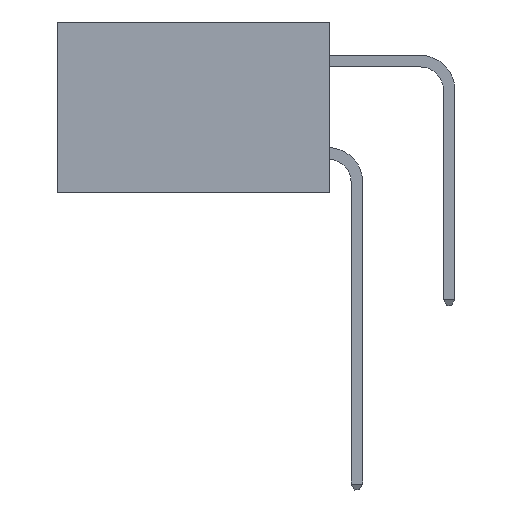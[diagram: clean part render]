
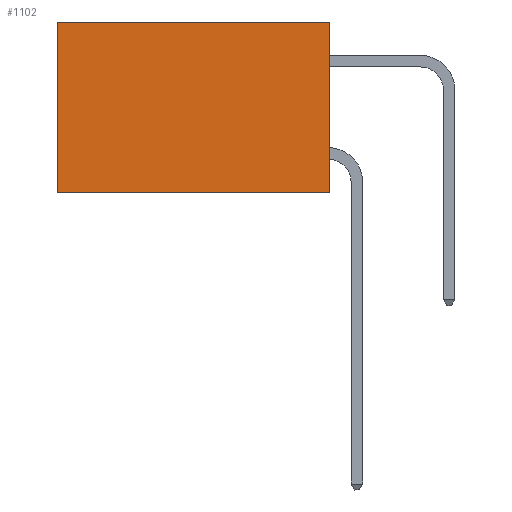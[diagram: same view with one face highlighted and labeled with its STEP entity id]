
A CAD part, left-side view. The second image highlights one B-rep face of the part: STEP entity #1102.
In plain terms, the highlighted planar face has unit normal (-1, 0, 0).
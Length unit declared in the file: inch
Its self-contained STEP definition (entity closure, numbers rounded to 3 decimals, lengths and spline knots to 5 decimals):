
#195 = AXIS2_PLACEMENT_3D ( 'NONE', #9011, #692, #2740 ) ;
#692 = DIRECTION ( 'NONE',  ( 1., 0., 0. ) ) ;
#1022 = DIRECTION ( 'NONE',  ( 0., 0., -1. ) ) ;
#1102 = ADVANCED_FACE ( 'NONE', ( #3993 ), #2985, .F. ) ;
#1484 = CARTESIAN_POINT ( 'NONE',  ( 0.277, 0.59, -0.37 ) ) ;
#1709 = DIRECTION ( 'NONE',  ( 0., 1., 0. ) ) ;
#2141 = CARTESIAN_POINT ( 'NONE',  ( 0.277, 0., 0. ) ) ;
#2303 = LINE ( 'NONE', #5238, #6686 ) ;
#2310 = VERTEX_POINT ( 'NONE', #2141 ) ;
#2450 = VERTEX_POINT ( 'NONE', #1484 ) ;
#2740 = DIRECTION ( 'NONE',  ( 0., 0., -1. ) ) ;
#2827 = CARTESIAN_POINT ( 'NONE',  ( 0.277, 0., 0. ) ) ;
#2985 = PLANE ( 'NONE',  #195 ) ;
#3219 = LINE ( 'NONE', #6325, #5651 ) ;
#3993 = FACE_OUTER_BOUND ( 'NONE', #5499, .T. ) ;
#5151 = CARTESIAN_POINT ( 'NONE',  ( 0.277, 0., -0.37 ) ) ;
#5194 = EDGE_CURVE ( 'NONE', #7130, #2450, #7757, .T. ) ;
#5238 = CARTESIAN_POINT ( 'NONE',  ( 0.277, 0., -0.37 ) ) ;
#5499 = EDGE_LOOP ( 'NONE', ( #8539, #8548, #8557, #8565 ) ) ;
#5651 = VECTOR ( 'NONE', #1022, 39.37008 ) ;
#6130 = EDGE_CURVE ( 'NONE', #8331, #2450, #2303, .T. ) ;
#6174 = EDGE_CURVE ( 'NONE', #2310, #8331, #3219, .T. ) ;
#6242 = EDGE_CURVE ( 'NONE', #2310, #7130, #6984, .T. ) ;
#6325 = CARTESIAN_POINT ( 'NONE',  ( 0.277, 0., -0.37 ) ) ;
#6429 = DIRECTION ( 'NONE',  ( 0., 1., 0. ) ) ;
#6563 = DIRECTION ( 'NONE',  ( 0., 0., -1. ) ) ;
#6686 = VECTOR ( 'NONE', #1709, 39.37008 ) ;
#6984 = LINE ( 'NONE', #2827, #8720 ) ;
#7130 = VERTEX_POINT ( 'NONE', #7728 ) ;
#7728 = CARTESIAN_POINT ( 'NONE',  ( 0.277, 0.59, 0. ) ) ;
#7757 = LINE ( 'NONE', #10002, #9497 ) ;
#8331 = VERTEX_POINT ( 'NONE', #5151 ) ;
#8539 = ORIENTED_EDGE ( 'NONE', *, *, #5194, .T. ) ;
#8548 = ORIENTED_EDGE ( 'NONE', *, *, #6130, .F. ) ;
#8557 = ORIENTED_EDGE ( 'NONE', *, *, #6174, .F. ) ;
#8565 = ORIENTED_EDGE ( 'NONE', *, *, #6242, .T. ) ;
#8720 = VECTOR ( 'NONE', #6429, 39.37008 ) ;
#9011 = CARTESIAN_POINT ( 'NONE',  ( 0.277, 0., -0.37 ) ) ;
#9497 = VECTOR ( 'NONE', #6563, 39.37008 ) ;
#10002 = CARTESIAN_POINT ( 'NONE',  ( 0.277, 0.59, -0.37 ) ) ;
